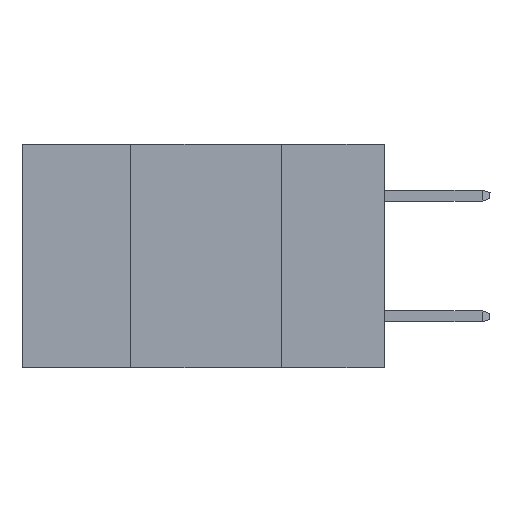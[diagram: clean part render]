
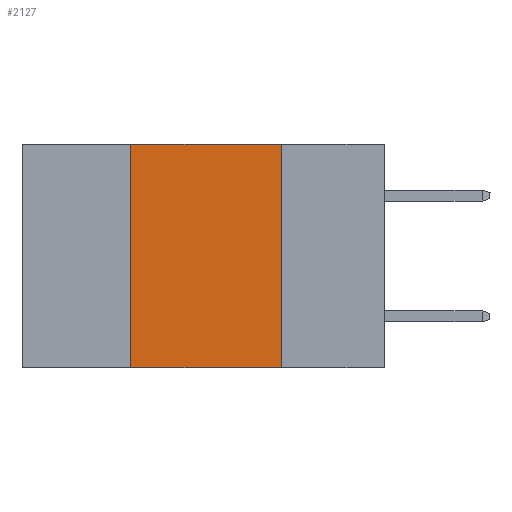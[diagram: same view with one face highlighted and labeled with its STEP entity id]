
A CAD part, left-side view. The second image highlights one B-rep face of the part: STEP entity #2127.
In plain terms, the highlighted planar face has unit normal (-1, 0, 0).
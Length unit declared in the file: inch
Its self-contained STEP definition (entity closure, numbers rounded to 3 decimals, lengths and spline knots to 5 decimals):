
#534 = CARTESIAN_POINT ( 'NONE',  ( 0., 0.6, 0. ) ) ;
#1044 = CARTESIAN_POINT ( 'NONE',  ( 0., 0.42, -0.37 ) ) ;
#1997 = DIRECTION ( 'NONE',  ( 0., -1., 0. ) ) ;
#2127 = ADVANCED_FACE ( 'NONE', ( #15670 ), #16585, .F. ) ;
#2196 = CARTESIAN_POINT ( 'NONE',  ( 0., 0.17, -0.37 ) ) ;
#2292 = DIRECTION ( 'NONE',  ( 1., 0., 0. ) ) ;
#2344 = DIRECTION ( 'NONE',  ( 0., 0., -1. ) ) ;
#2904 = LINE ( 'NONE', #14282, #15729 ) ;
#3274 = EDGE_CURVE ( 'NONE', #11322, #20305, #18058, .T. ) ;
#3303 = DIRECTION ( 'NONE',  ( 0., 0., -1. ) ) ;
#3310 = VERTEX_POINT ( 'NONE', #4845 ) ;
#4190 = VECTOR ( 'NONE', #2344, 39.37008 ) ;
#4845 = CARTESIAN_POINT ( 'NONE',  ( 0., 0.42, -0.37 ) ) ;
#5692 = CARTESIAN_POINT ( 'NONE',  ( 0., 0.17, -0.37 ) ) ;
#6270 = CARTESIAN_POINT ( 'NONE',  ( 0., 0.17, 0. ) ) ;
#8096 = DIRECTION ( 'NONE',  ( 0., 0., 1. ) ) ;
#10191 = VECTOR ( 'NONE', #13947, 39.37008 ) ;
#11322 = VERTEX_POINT ( 'NONE', #6270 ) ;
#12724 = ORIENTED_EDGE ( 'NONE', *, *, #21226, .F. ) ;
#12755 = EDGE_LOOP ( 'NONE', ( #14759, #15210, #12724, #18863 ) ) ;
#13736 = LINE ( 'NONE', #22562, #10191 ) ;
#13947 = DIRECTION ( 'NONE',  ( 0., -1., 0. ) ) ;
#14282 = CARTESIAN_POINT ( 'NONE',  ( 0., 0.6, -0.37 ) ) ;
#14759 = ORIENTED_EDGE ( 'NONE', *, *, #3274, .F. ) ;
#14804 = VECTOR ( 'NONE', #8096, 39.37008 ) ;
#15210 = ORIENTED_EDGE ( 'NONE', *, *, #20787, .F. ) ;
#15670 = FACE_OUTER_BOUND ( 'NONE', #12755, .T. ) ;
#15729 = VECTOR ( 'NONE', #1997, 39.37008 ) ;
#16585 = PLANE ( 'NONE',  #21947 ) ;
#16971 = CARTESIAN_POINT ( 'NONE',  ( 0., 0.42, 0. ) ) ;
#18058 = LINE ( 'NONE', #2196, #4190 ) ;
#18300 = LINE ( 'NONE', #1044, #14804 ) ;
#18450 = EDGE_CURVE ( 'NONE', #3310, #20305, #2904, .T. ) ;
#18863 = ORIENTED_EDGE ( 'NONE', *, *, #18450, .T. ) ;
#20305 = VERTEX_POINT ( 'NONE', #5692 ) ;
#20637 = VERTEX_POINT ( 'NONE', #16971 ) ;
#20787 = EDGE_CURVE ( 'NONE', #20637, #11322, #13736, .T. ) ;
#21226 = EDGE_CURVE ( 'NONE', #3310, #20637, #18300, .T. ) ;
#21947 = AXIS2_PLACEMENT_3D ( 'NONE', #534, #2292, #3303 ) ;
#22562 = CARTESIAN_POINT ( 'NONE',  ( 0., 0.6, 0. ) ) ;
